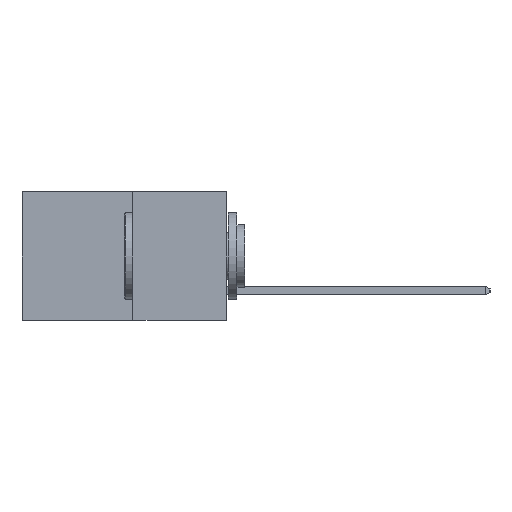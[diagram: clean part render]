
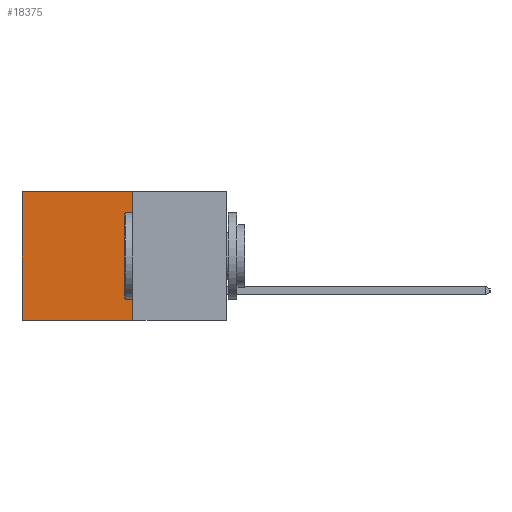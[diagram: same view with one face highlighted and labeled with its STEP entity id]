
A CAD part, left-side view. The second image highlights one B-rep face of the part: STEP entity #18375.
In plain terms, the highlighted planar face has unit normal (-1, 0, 0).
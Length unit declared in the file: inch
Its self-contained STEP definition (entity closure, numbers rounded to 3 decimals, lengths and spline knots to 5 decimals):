
#262 = DIRECTION ( 'NONE',  ( 0., 0., -1. ) ) ;
#403 = VERTEX_POINT ( 'NONE', #16784 ) ;
#1015 = EDGE_CURVE ( 'NONE', #16819, #403, #17062, .T. ) ;
#1100 = VECTOR ( 'NONE', #1778, 39.37008 ) ;
#1759 = DIRECTION ( 'NONE',  ( 1., 0., 0. ) ) ;
#1778 = DIRECTION ( 'NONE',  ( 0., 0., -1. ) ) ;
#2220 = CARTESIAN_POINT ( 'NONE',  ( 0.277, 0.59, -0.37 ) ) ;
#2778 = CARTESIAN_POINT ( 'NONE',  ( 0.277, 0.27, 0. ) ) ;
#3852 = AXIS2_PLACEMENT_3D ( 'NONE', #15644, #1759, #12658 ) ;
#4275 = VECTOR ( 'NONE', #4353, 39.37008 ) ;
#4353 = DIRECTION ( 'NONE',  ( 0., 1., 0. ) ) ;
#4455 = EDGE_CURVE ( 'NONE', #19083, #403, #19030, .T. ) ;
#4520 = ORIENTED_EDGE ( 'NONE', *, *, #8557, .F. ) ;
#5032 = CARTESIAN_POINT ( 'NONE',  ( 0.277, 0.27, -0.37 ) ) ;
#5567 = CARTESIAN_POINT ( 'NONE',  ( 0.277, 0.59, 0. ) ) ;
#6921 = ORIENTED_EDGE ( 'NONE', *, *, #1015, .T. ) ;
#7213 = VERTEX_POINT ( 'NONE', #8862 ) ;
#7290 = EDGE_CURVE ( 'NONE', #7213, #16819, #8520, .T. ) ;
#8520 = LINE ( 'NONE', #2778, #4275 ) ;
#8557 = EDGE_CURVE ( 'NONE', #7213, #19083, #9421, .T. ) ;
#8570 = CARTESIAN_POINT ( 'NONE',  ( 0.277, 0.27, -0.37 ) ) ;
#8862 = CARTESIAN_POINT ( 'NONE',  ( 0.277, 0.27, 0. ) ) ;
#9421 = LINE ( 'NONE', #5032, #17002 ) ;
#9607 = ORIENTED_EDGE ( 'NONE', *, *, #7290, .T. ) ;
#10094 = DIRECTION ( 'NONE',  ( 0., 1., 0. ) ) ;
#11123 = PLANE ( 'NONE',  #3852 ) ;
#11528 = ORIENTED_EDGE ( 'NONE', *, *, #4455, .F. ) ;
#12658 = DIRECTION ( 'NONE',  ( 0., 0., -1. ) ) ;
#15409 = EDGE_LOOP ( 'NONE', ( #6921, #11528, #4520, #9607 ) ) ;
#15644 = CARTESIAN_POINT ( 'NONE',  ( 0.277, 0.27, -0.37 ) ) ;
#16784 = CARTESIAN_POINT ( 'NONE',  ( 0.277, 0.59, -0.37 ) ) ;
#16819 = VERTEX_POINT ( 'NONE', #5567 ) ;
#17002 = VECTOR ( 'NONE', #262, 39.37008 ) ;
#17062 = LINE ( 'NONE', #2220, #1100 ) ;
#18035 = FACE_OUTER_BOUND ( 'NONE', #15409, .T. ) ;
#18375 = ADVANCED_FACE ( 'NONE', ( #18035 ), #11123, .F. ) ;
#18559 = VECTOR ( 'NONE', #10094, 39.37008 ) ;
#18942 = CARTESIAN_POINT ( 'NONE',  ( 0.277, 0.27, -0.37 ) ) ;
#19030 = LINE ( 'NONE', #8570, #18559 ) ;
#19083 = VERTEX_POINT ( 'NONE', #18942 ) ;
